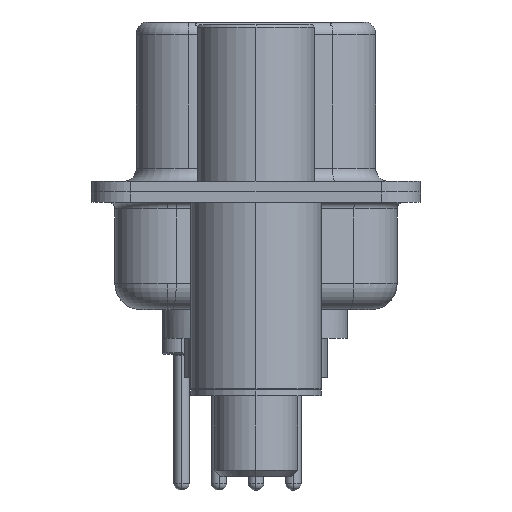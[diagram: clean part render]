
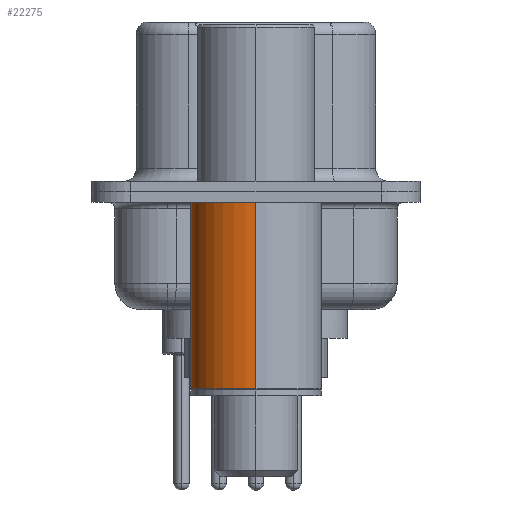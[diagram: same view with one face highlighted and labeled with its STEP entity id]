
A CAD part, left-side view. The second image highlights one B-rep face of the part: STEP entity #22275.
In plain terms, the highlighted cylindrical face has radius 2.5 mm (diameter 5 mm), a partial arc.
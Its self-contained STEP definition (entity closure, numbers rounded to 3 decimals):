
#2421 = ORIENTED_EDGE ( 'NONE', *, *, #18503, .F. ) ;
#2598 = CARTESIAN_POINT ( 'NONE',  ( 0., 0., -0.4 ) ) ;
#3601 = AXIS2_PLACEMENT_3D ( 'NONE', #2598, #17301, #4689 ) ;
#4227 = AXIS2_PLACEMENT_3D ( 'NONE', #25867, #21574, #16190 ) ;
#4629 = LINE ( 'NONE', #25755, #15124 ) ;
#4689 = DIRECTION ( 'NONE',  ( 1., 0., 0. ) ) ;
#4952 = VERTEX_POINT ( 'NONE', #26091 ) ;
#5211 = EDGE_CURVE ( 'NONE', #13930, #4952, #4629, .T. ) ;
#5702 = ORIENTED_EDGE ( 'NONE', *, *, #6099, .T. ) ;
#6099 = EDGE_CURVE ( 'NONE', #21704, #13930, #13438, .T. ) ;
#6358 = DIRECTION ( 'NONE',  ( 0., 0., 1. ) ) ;
#7602 = FACE_OUTER_BOUND ( 'NONE', #7728, .T. ) ;
#7728 = EDGE_LOOP ( 'NONE', ( #5702, #27272, #23012, #2421 ) ) ;
#10417 = DIRECTION ( 'NONE',  ( 0., 0., 1. ) ) ;
#11049 = CARTESIAN_POINT ( 'NONE',  ( 2.5, 0., -0.4 ) ) ;
#11268 = VECTOR ( 'NONE', #6358, 1000. ) ;
#12441 = DIRECTION ( 'NONE',  ( 1., 0., 0. ) ) ;
#13438 = CIRCLE ( 'NONE', #4227, 2.5 ) ;
#13930 = VERTEX_POINT ( 'NONE', #26248 ) ;
#14684 = VERTEX_POINT ( 'NONE', #11049 ) ;
#14896 = CIRCLE ( 'NONE', #3601, 2.5 ) ;
#15124 = VECTOR ( 'NONE', #10417, 1000. ) ;
#16190 = DIRECTION ( 'NONE',  ( 1., 0., 0. ) ) ;
#16919 = LINE ( 'NONE', #18946, #11268 ) ;
#17301 = DIRECTION ( 'NONE',  ( 0., 0., 1. ) ) ;
#18115 = CYLINDRICAL_SURFACE ( 'NONE', #22559, 2.5 ) ;
#18503 = EDGE_CURVE ( 'NONE', #21704, #14684, #16919, .T. ) ;
#18621 = EDGE_CURVE ( 'NONE', #14684, #4952, #14896, .T. ) ;
#18946 = CARTESIAN_POINT ( 'NONE',  ( 2.5, 0., 0.581 ) ) ;
#21574 = DIRECTION ( 'NONE',  ( 0., 0., 1. ) ) ;
#21704 = VERTEX_POINT ( 'NONE', #27379 ) ;
#22275 = ADVANCED_FACE ( 'NONE', ( #7602 ), #18115, .T. ) ;
#22559 = AXIS2_PLACEMENT_3D ( 'NONE', #25212, #23046, #12441 ) ;
#23012 = ORIENTED_EDGE ( 'NONE', *, *, #18621, .F. ) ;
#23046 = DIRECTION ( 'NONE',  ( 0., 0., 1. ) ) ;
#25212 = CARTESIAN_POINT ( 'NONE',  ( 0., 0., 0.581 ) ) ;
#25755 = CARTESIAN_POINT ( 'NONE',  ( -2.5, 0., 0.581 ) ) ;
#25867 = CARTESIAN_POINT ( 'NONE',  ( 0., 0., -7.525 ) ) ;
#26091 = CARTESIAN_POINT ( 'NONE',  ( -2.5, 0., -0.4 ) ) ;
#26248 = CARTESIAN_POINT ( 'NONE',  ( -2.5, 0., -7.525 ) ) ;
#27272 = ORIENTED_EDGE ( 'NONE', *, *, #5211, .T. ) ;
#27379 = CARTESIAN_POINT ( 'NONE',  ( 2.5, 0., -7.525 ) ) ;
